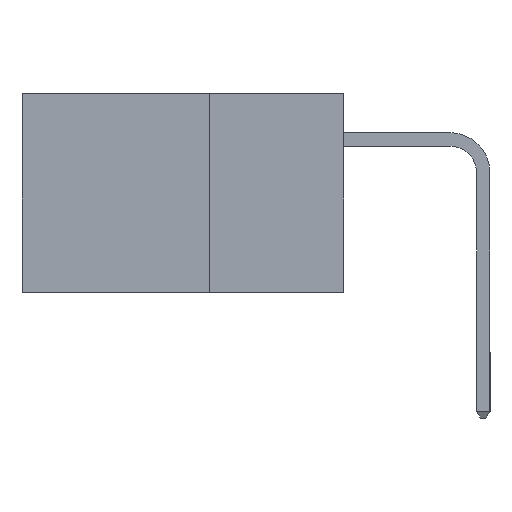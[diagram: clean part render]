
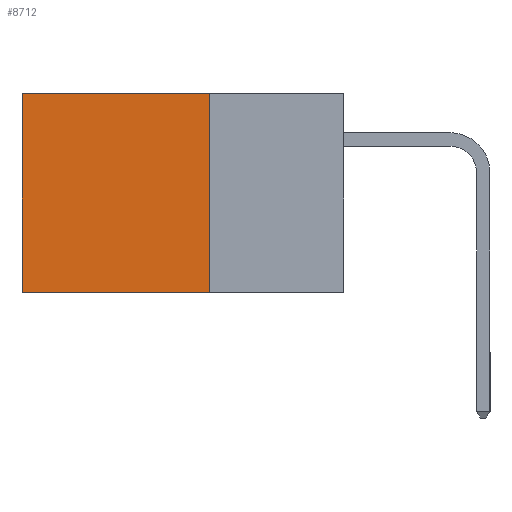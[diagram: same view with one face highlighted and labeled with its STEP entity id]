
A CAD part, left-side view. The second image highlights one B-rep face of the part: STEP entity #8712.
In plain terms, the highlighted planar face has unit normal (-1, 0, 0).
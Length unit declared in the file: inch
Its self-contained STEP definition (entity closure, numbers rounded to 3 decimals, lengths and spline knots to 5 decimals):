
#453 = LINE ( 'NONE', #817, #9835 ) ;
#626 = EDGE_LOOP ( 'NONE', ( #6394, #7679, #1289, #4906 ) ) ;
#817 = CARTESIAN_POINT ( 'NONE',  ( 0.298, 0.25, 0. ) ) ;
#1289 = ORIENTED_EDGE ( 'NONE', *, *, #9669, .F. ) ;
#1325 = VERTEX_POINT ( 'NONE', #6167 ) ;
#1995 = DIRECTION ( 'NONE',  ( 1., 0., 0. ) ) ;
#2221 = LINE ( 'NONE', #3355, #9488 ) ;
#2525 = DIRECTION ( 'NONE',  ( 0., 1., 0. ) ) ;
#2628 = CARTESIAN_POINT ( 'NONE',  ( 0.298, 0.6, 0. ) ) ;
#3072 = LINE ( 'NONE', #2628, #4732 ) ;
#3168 = VERTEX_POINT ( 'NONE', #8289 ) ;
#3355 = CARTESIAN_POINT ( 'NONE',  ( 0.298, 0.25, 0. ) ) ;
#3382 = EDGE_CURVE ( 'NONE', #1325, #7333, #4955, .T. ) ;
#3388 = CARTESIAN_POINT ( 'NONE',  ( 0.298, 0.25, 0. ) ) ;
#3893 = VECTOR ( 'NONE', #4693, 39.37008 ) ;
#4501 = FACE_OUTER_BOUND ( 'NONE', #626, .T. ) ;
#4693 = DIRECTION ( 'NONE',  ( 0., 1., 0. ) ) ;
#4732 = VECTOR ( 'NONE', #6365, 39.37008 ) ;
#4906 = ORIENTED_EDGE ( 'NONE', *, *, #9274, .T. ) ;
#4955 = LINE ( 'NONE', #7491, #3893 ) ;
#5655 = VERTEX_POINT ( 'NONE', #3388 ) ;
#6137 = DIRECTION ( 'NONE',  ( 0., 0., -1. ) ) ;
#6167 = CARTESIAN_POINT ( 'NONE',  ( 0.298, 0.25, -0.37 ) ) ;
#6365 = DIRECTION ( 'NONE',  ( 0., 0., -1. ) ) ;
#6394 = ORIENTED_EDGE ( 'NONE', *, *, #9235, .T. ) ;
#6538 = CARTESIAN_POINT ( 'NONE',  ( 0.298, 0.25, 0. ) ) ;
#7282 = PLANE ( 'NONE',  #7985 ) ;
#7313 = DIRECTION ( 'NONE',  ( 0., 0., -1. ) ) ;
#7333 = VERTEX_POINT ( 'NONE', #8677 ) ;
#7491 = CARTESIAN_POINT ( 'NONE',  ( 0.298, 0.25, -0.37 ) ) ;
#7679 = ORIENTED_EDGE ( 'NONE', *, *, #3382, .F. ) ;
#7985 = AXIS2_PLACEMENT_3D ( 'NONE', #6538, #1995, #7313 ) ;
#8289 = CARTESIAN_POINT ( 'NONE',  ( 0.298, 0.6, 0. ) ) ;
#8677 = CARTESIAN_POINT ( 'NONE',  ( 0.298, 0.6, -0.37 ) ) ;
#8712 = ADVANCED_FACE ( 'NONE', ( #4501 ), #7282, .F. ) ;
#9235 = EDGE_CURVE ( 'NONE', #3168, #7333, #3072, .T. ) ;
#9274 = EDGE_CURVE ( 'NONE', #5655, #3168, #2221, .T. ) ;
#9488 = VECTOR ( 'NONE', #2525, 39.37008 ) ;
#9669 = EDGE_CURVE ( 'NONE', #5655, #1325, #453, .T. ) ;
#9835 = VECTOR ( 'NONE', #6137, 39.37008 ) ;
